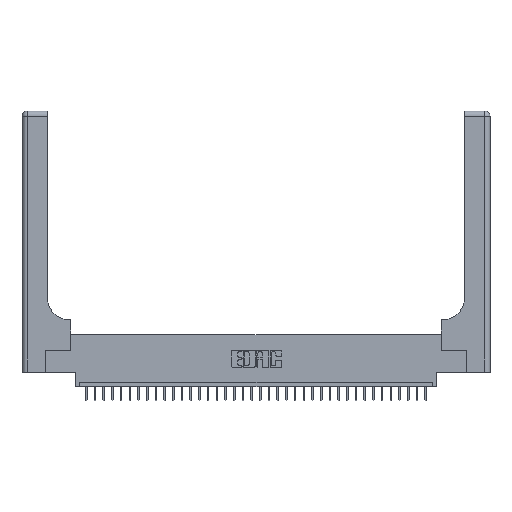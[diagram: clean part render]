
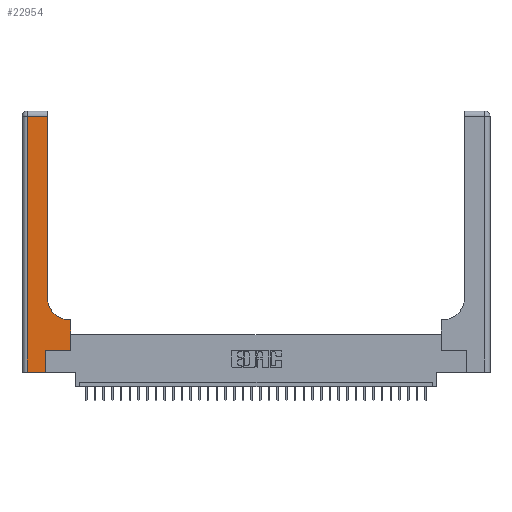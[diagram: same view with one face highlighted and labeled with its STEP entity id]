
A CAD part, top view. The second image highlights one B-rep face of the part: STEP entity #22954.
In plain terms, the highlighted planar face has unit normal (0, 0, 1).
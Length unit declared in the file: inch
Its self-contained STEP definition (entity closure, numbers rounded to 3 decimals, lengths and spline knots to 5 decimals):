
#1258 = LINE ( 'NONE', #19960, #29720 ) ;
#1536 = EDGE_CURVE ( 'NONE', #29732, #4514, #1258, .T. ) ;
#1799 = ORIENTED_EDGE ( 'NONE', *, *, #1536, .T. ) ;
#2242 = EDGE_CURVE ( 'NONE', #29994, #6213, #2482, .T. ) ;
#2482 = CIRCLE ( 'NONE', #15084, 0.25 ) ;
#3030 = DIRECTION ( 'NONE',  ( -1., 0., 0. ) ) ;
#3240 = CARTESIAN_POINT ( 'NONE',  ( 0.5415, 0.85, 0.37 ) ) ;
#3670 = VECTOR ( 'NONE', #18281, 39.37008 ) ;
#3980 = ORIENTED_EDGE ( 'NONE', *, *, #12172, .T. ) ;
#4514 = VERTEX_POINT ( 'NONE', #7152 ) ;
#4981 = VECTOR ( 'NONE', #29265, 39.37008 ) ;
#5103 = VECTOR ( 'NONE', #9064, 39.37008 ) ;
#5722 = CARTESIAN_POINT ( 'NONE',  ( 0.5415, 0.6, 0.37 ) ) ;
#6213 = VERTEX_POINT ( 'NONE', #34058 ) ;
#6287 = VERTEX_POINT ( 'NONE', #17123 ) ;
#7152 = CARTESIAN_POINT ( 'NONE',  ( 0.5585, 0.6, 0.37 ) ) ;
#7357 = VERTEX_POINT ( 'NONE', #14711 ) ;
#7679 = VECTOR ( 'NONE', #31380, 39.37008 ) ;
#8712 = AXIS2_PLACEMENT_3D ( 'NONE', #11212, #30533, #3030 ) ;
#8744 = CARTESIAN_POINT ( 'NONE',  ( 0.2915, 2.94, 0.37 ) ) ;
#9064 = DIRECTION ( 'NONE',  ( 0., 1., 0. ) ) ;
#10998 = LINE ( 'NONE', #21211, #3670 ) ;
#11155 = ORIENTED_EDGE ( 'NONE', *, *, #32325, .T. ) ;
#11212 = CARTESIAN_POINT ( 'NONE',  ( 0., 3., 0.37 ) ) ;
#12172 = EDGE_CURVE ( 'NONE', #20199, #23080, #34942, .T. ) ;
#13039 = CARTESIAN_POINT ( 'NONE',  ( 0.2915, 0.6, 0.37 ) ) ;
#13088 = EDGE_CURVE ( 'NONE', #6213, #20199, #21441, .T. ) ;
#13280 = DIRECTION ( 'NONE',  ( -1., 0., 0. ) ) ;
#13339 = EDGE_CURVE ( 'NONE', #6287, #7357, #10998, .T. ) ;
#13564 = CARTESIAN_POINT ( 'NONE',  ( 0.269, 0.25, 0.37 ) ) ;
#13650 = ORIENTED_EDGE ( 'NONE', *, *, #19424, .T. ) ;
#14462 = LINE ( 'NONE', #13564, #4981 ) ;
#14711 = CARTESIAN_POINT ( 'NONE',  ( 0.269, 0., 0.37 ) ) ;
#14856 = ORIENTED_EDGE ( 'NONE', *, *, #17253, .T. ) ;
#15084 = AXIS2_PLACEMENT_3D ( 'NONE', #3240, #22803, #29393 ) ;
#15602 = ORIENTED_EDGE ( 'NONE', *, *, #13339, .T. ) ;
#16269 = VECTOR ( 'NONE', #29017, 39.37008 ) ;
#17123 = CARTESIAN_POINT ( 'NONE',  ( 0.06, 0., 0.37 ) ) ;
#17253 = EDGE_CURVE ( 'NONE', #7357, #33078, #32351, .T. ) ;
#17761 = DIRECTION ( 'NONE',  ( 0., -1., 0. ) ) ;
#17876 = VECTOR ( 'NONE', #13280, 39.37008 ) ;
#17887 = CARTESIAN_POINT ( 'NONE',  ( 0.06, 3., 0.37 ) ) ;
#17908 = EDGE_LOOP ( 'NONE', ( #30847, #3980, #22715, #15602, #14856, #13650, #1799, #11155, #31709 ) ) ;
#17962 = LINE ( 'NONE', #17887, #30904 ) ;
#18116 = EDGE_CURVE ( 'NONE', #23080, #6287, #17962, .T. ) ;
#18281 = DIRECTION ( 'NONE',  ( 1., 0., 0. ) ) ;
#18346 = LINE ( 'NONE', #13039, #17876 ) ;
#19424 = EDGE_CURVE ( 'NONE', #33078, #29732, #14462, .T. ) ;
#19643 = CARTESIAN_POINT ( 'NONE',  ( 0.269, 0.25, 0.37 ) ) ;
#19960 = CARTESIAN_POINT ( 'NONE',  ( 0.5585, 0.25, 0.37 ) ) ;
#20193 = CARTESIAN_POINT ( 'NONE',  ( 0.269, 0., 0.37 ) ) ;
#20199 = VERTEX_POINT ( 'NONE', #8744 ) ;
#20789 = CARTESIAN_POINT ( 'NONE',  ( 0.06, 2.94, 0.37 ) ) ;
#21211 = CARTESIAN_POINT ( 'NONE',  ( 0., 0., 0.37 ) ) ;
#21441 = LINE ( 'NONE', #23465, #16269 ) ;
#22715 = ORIENTED_EDGE ( 'NONE', *, *, #18116, .T. ) ;
#22742 = DIRECTION ( 'NONE',  ( 0., 1., 0. ) ) ;
#22803 = DIRECTION ( 'NONE',  ( 0., 0., -1. ) ) ;
#22954 = ADVANCED_FACE ( 'NONE', ( #26521 ), #27783, .F. ) ;
#23080 = VERTEX_POINT ( 'NONE', #20789 ) ;
#23465 = CARTESIAN_POINT ( 'NONE',  ( 0.2915, 3., 0.37 ) ) ;
#26521 = FACE_OUTER_BOUND ( 'NONE', #17908, .T. ) ;
#27783 = PLANE ( 'NONE',  #8712 ) ;
#29017 = DIRECTION ( 'NONE',  ( 0., 1., 0. ) ) ;
#29265 = DIRECTION ( 'NONE',  ( 1., 0., 0. ) ) ;
#29393 = DIRECTION ( 'NONE',  ( 1., 0., 0. ) ) ;
#29720 = VECTOR ( 'NONE', #22742, 39.37008 ) ;
#29732 = VERTEX_POINT ( 'NONE', #35386 ) ;
#29994 = VERTEX_POINT ( 'NONE', #5722 ) ;
#30533 = DIRECTION ( 'NONE',  ( 0., 0., -1. ) ) ;
#30847 = ORIENTED_EDGE ( 'NONE', *, *, #13088, .T. ) ;
#30904 = VECTOR ( 'NONE', #17761, 39.37008 ) ;
#31380 = DIRECTION ( 'NONE',  ( -1., 0., 0. ) ) ;
#31514 = CARTESIAN_POINT ( 'NONE',  ( 0., 2.94, 0.37 ) ) ;
#31709 = ORIENTED_EDGE ( 'NONE', *, *, #2242, .T. ) ;
#32325 = EDGE_CURVE ( 'NONE', #4514, #29994, #18346, .T. ) ;
#32351 = LINE ( 'NONE', #20193, #5103 ) ;
#33078 = VERTEX_POINT ( 'NONE', #19643 ) ;
#34058 = CARTESIAN_POINT ( 'NONE',  ( 0.2915, 0.85, 0.37 ) ) ;
#34942 = LINE ( 'NONE', #31514, #7679 ) ;
#35386 = CARTESIAN_POINT ( 'NONE',  ( 0.5585, 0.25, 0.37 ) ) ;
